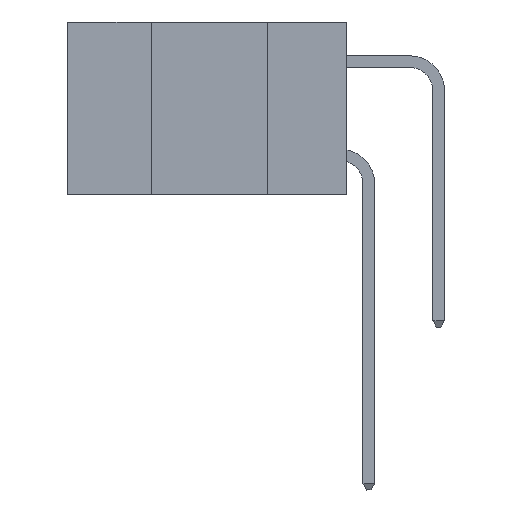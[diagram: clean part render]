
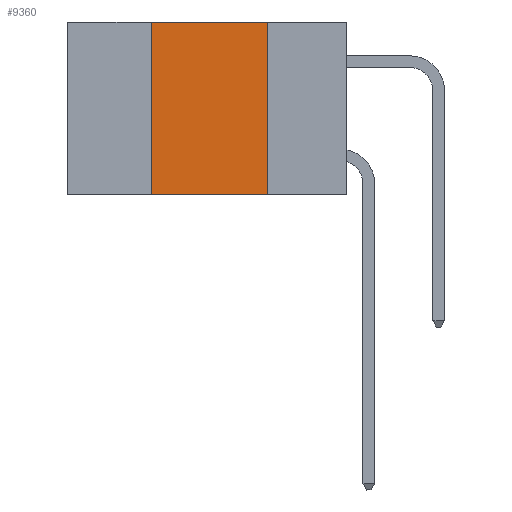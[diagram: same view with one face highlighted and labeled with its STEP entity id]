
A CAD part, left-side view. The second image highlights one B-rep face of the part: STEP entity #9360.
In plain terms, the highlighted planar face has unit normal (-1, 0, 0).
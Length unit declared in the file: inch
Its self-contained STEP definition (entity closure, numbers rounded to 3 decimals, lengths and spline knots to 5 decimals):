
#51 = ORIENTED_EDGE ( 'NONE', *, *, #21837, .F. ) ;
#179 = VERTEX_POINT ( 'NONE', #24603 ) ;
#1307 = EDGE_CURVE ( 'NONE', #1688, #179, #21441, .T. ) ;
#1688 = VERTEX_POINT ( 'NONE', #24217 ) ;
#1923 = ORIENTED_EDGE ( 'NONE', *, *, #4225, .F. ) ;
#2990 = LINE ( 'NONE', #7120, #11473 ) ;
#4225 = EDGE_CURVE ( 'NONE', #1688, #23580, #2990, .T. ) ;
#5726 = EDGE_CURVE ( 'NONE', #7875, #179, #12899, .T. ) ;
#6185 = CARTESIAN_POINT ( 'NONE',  ( 0., 0.17, 0. ) ) ;
#7120 = CARTESIAN_POINT ( 'NONE',  ( 0., 0.42, 0. ) ) ;
#7179 = VECTOR ( 'NONE', #21430, 39.37008 ) ;
#7380 = EDGE_LOOP ( 'NONE', ( #23841, #51, #1923, #7738 ) ) ;
#7738 = ORIENTED_EDGE ( 'NONE', *, *, #1307, .T. ) ;
#7875 = VERTEX_POINT ( 'NONE', #16221 ) ;
#8563 = DIRECTION ( 'NONE',  ( 0., -1., 0. ) ) ;
#9326 = DIRECTION ( 'NONE',  ( 1., 0., 0. ) ) ;
#9360 = ADVANCED_FACE ( 'NONE', ( #11410 ), #16987, .F. ) ;
#11410 = FACE_OUTER_BOUND ( 'NONE', #7380, .T. ) ;
#11473 = VECTOR ( 'NONE', #16704, 39.37008 ) ;
#11660 = VECTOR ( 'NONE', #23641, 39.37008 ) ;
#11944 = VECTOR ( 'NONE', #8563, 39.37008 ) ;
#12899 = LINE ( 'NONE', #6185, #7179 ) ;
#14959 = CARTESIAN_POINT ( 'NONE',  ( 0., 0.42, 0. ) ) ;
#16221 = CARTESIAN_POINT ( 'NONE',  ( 0., 0.17, 0. ) ) ;
#16704 = DIRECTION ( 'NONE',  ( 0., 0., 1. ) ) ;
#16745 = CARTESIAN_POINT ( 'NONE',  ( 0., 0.6, -0.37 ) ) ;
#16874 = AXIS2_PLACEMENT_3D ( 'NONE', #20747, #9326, #22643 ) ;
#16987 = PLANE ( 'NONE',  #16874 ) ;
#20747 = CARTESIAN_POINT ( 'NONE',  ( 0., 0.6, 0. ) ) ;
#21167 = LINE ( 'NONE', #21710, #11660 ) ;
#21430 = DIRECTION ( 'NONE',  ( 0., 0., -1. ) ) ;
#21441 = LINE ( 'NONE', #16745, #11944 ) ;
#21710 = CARTESIAN_POINT ( 'NONE',  ( 0., 0.6, 0. ) ) ;
#21837 = EDGE_CURVE ( 'NONE', #23580, #7875, #21167, .T. ) ;
#22643 = DIRECTION ( 'NONE',  ( 0., 0., -1. ) ) ;
#23580 = VERTEX_POINT ( 'NONE', #14959 ) ;
#23641 = DIRECTION ( 'NONE',  ( 0., -1., 0. ) ) ;
#23841 = ORIENTED_EDGE ( 'NONE', *, *, #5726, .F. ) ;
#24217 = CARTESIAN_POINT ( 'NONE',  ( 0., 0.42, -0.37 ) ) ;
#24603 = CARTESIAN_POINT ( 'NONE',  ( 0., 0.17, -0.37 ) ) ;
